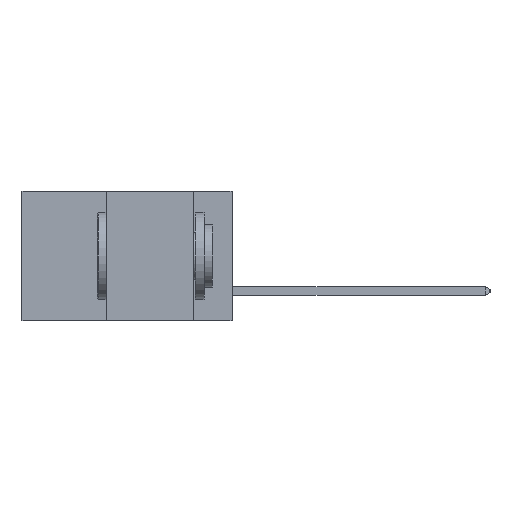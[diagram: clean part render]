
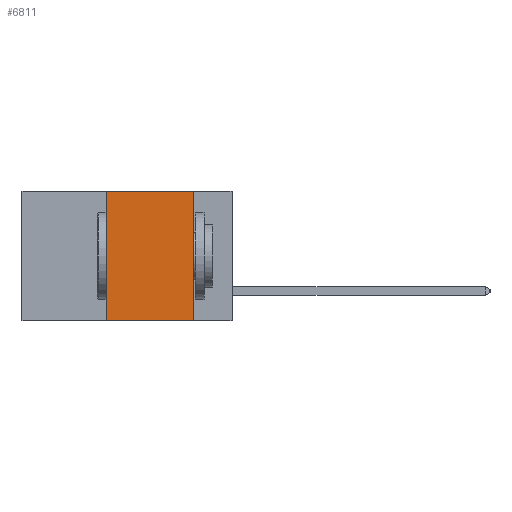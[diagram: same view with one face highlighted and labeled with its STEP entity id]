
A CAD part, left-side view. The second image highlights one B-rep face of the part: STEP entity #6811.
In plain terms, the highlighted planar face has unit normal (-1, 0, 0).
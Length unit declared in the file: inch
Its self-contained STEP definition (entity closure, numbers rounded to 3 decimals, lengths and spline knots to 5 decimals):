
#333 = LINE ( 'NONE', #10903, #10601 ) ;
#543 = DIRECTION ( 'NONE',  ( 1., 0., 0. ) ) ;
#973 = CARTESIAN_POINT ( 'NONE',  ( 0., 0.36, 0. ) ) ;
#1533 = EDGE_CURVE ( 'NONE', #7730, #14581, #10134, .T. ) ;
#2932 = CARTESIAN_POINT ( 'NONE',  ( 0., 0.6, 0. ) ) ;
#3818 = VERTEX_POINT ( 'NONE', #14987 ) ;
#4300 = ORIENTED_EDGE ( 'NONE', *, *, #14156, .F. ) ;
#5617 = ORIENTED_EDGE ( 'NONE', *, *, #24861, .F. ) ;
#6157 = CARTESIAN_POINT ( 'NONE',  ( 0., 0.11, -0.37 ) ) ;
#6655 = CARTESIAN_POINT ( 'NONE',  ( 0., 0.6, 0. ) ) ;
#6811 = ADVANCED_FACE ( 'NONE', ( #11140 ), #24820, .F. ) ;
#7730 = VERTEX_POINT ( 'NONE', #19626 ) ;
#10134 = LINE ( 'NONE', #20989, #10763 ) ;
#10317 = DIRECTION ( 'NONE',  ( 0., 0., 1. ) ) ;
#10601 = VECTOR ( 'NONE', #18934, 39.37008 ) ;
#10763 = VECTOR ( 'NONE', #20987, 39.37008 ) ;
#10903 = CARTESIAN_POINT ( 'NONE',  ( 0., 0.6, -0.37 ) ) ;
#11037 = ORIENTED_EDGE ( 'NONE', *, *, #25179, .T. ) ;
#11140 = FACE_OUTER_BOUND ( 'NONE', #17546, .T. ) ;
#11476 = VERTEX_POINT ( 'NONE', #973 ) ;
#13493 = VECTOR ( 'NONE', #10317, 39.37008 ) ;
#14156 = EDGE_CURVE ( 'NONE', #11476, #7730, #15548, .T. ) ;
#14581 = VERTEX_POINT ( 'NONE', #6157 ) ;
#14842 = DIRECTION ( 'NONE',  ( 0., 0., -1. ) ) ;
#14987 = CARTESIAN_POINT ( 'NONE',  ( 0., 0.36, -0.37 ) ) ;
#15548 = LINE ( 'NONE', #2932, #20258 ) ;
#17054 = DIRECTION ( 'NONE',  ( 0., -1., 0. ) ) ;
#17546 = EDGE_LOOP ( 'NONE', ( #25182, #4300, #5617, #11037 ) ) ;
#18331 = CARTESIAN_POINT ( 'NONE',  ( 0., 0.36, 0. ) ) ;
#18827 = LINE ( 'NONE', #18331, #13493 ) ;
#18934 = DIRECTION ( 'NONE',  ( 0., -1., 0. ) ) ;
#18945 = AXIS2_PLACEMENT_3D ( 'NONE', #6655, #543, #14842 ) ;
#19626 = CARTESIAN_POINT ( 'NONE',  ( 0., 0.11, 0. ) ) ;
#20258 = VECTOR ( 'NONE', #17054, 39.37008 ) ;
#20987 = DIRECTION ( 'NONE',  ( 0., 0., -1. ) ) ;
#20989 = CARTESIAN_POINT ( 'NONE',  ( 0., 0.11, 0. ) ) ;
#24820 = PLANE ( 'NONE',  #18945 ) ;
#24861 = EDGE_CURVE ( 'NONE', #3818, #11476, #18827, .T. ) ;
#25179 = EDGE_CURVE ( 'NONE', #3818, #14581, #333, .T. ) ;
#25182 = ORIENTED_EDGE ( 'NONE', *, *, #1533, .F. ) ;
